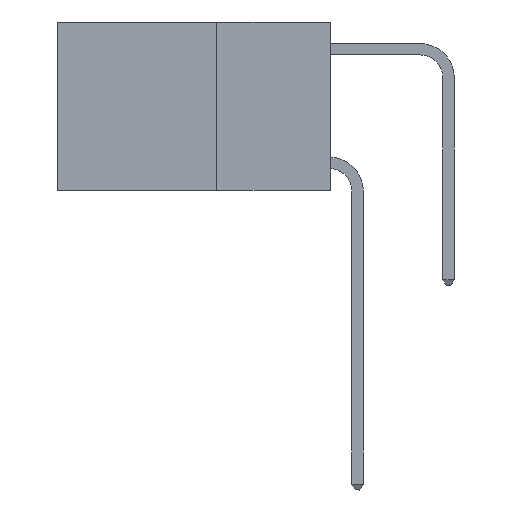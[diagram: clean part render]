
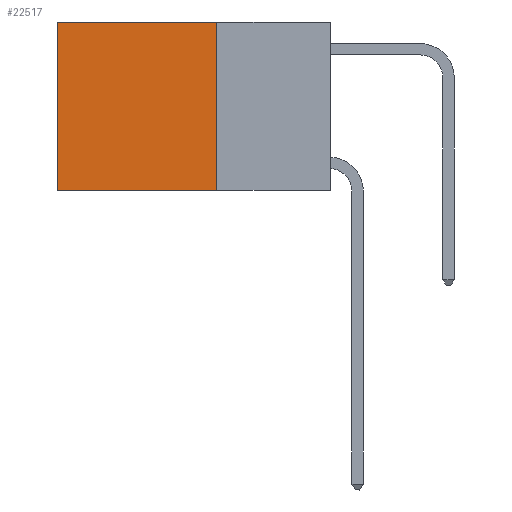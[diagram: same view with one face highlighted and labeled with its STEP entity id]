
A CAD part, left-side view. The second image highlights one B-rep face of the part: STEP entity #22517.
In plain terms, the highlighted planar face has unit normal (-1, 0, 0).
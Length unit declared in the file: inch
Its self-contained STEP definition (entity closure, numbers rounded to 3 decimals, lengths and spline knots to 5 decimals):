
#277 = CARTESIAN_POINT ( 'NONE',  ( 0.2625, 0.6, 0. ) ) ;
#510 = ORIENTED_EDGE ( 'NONE', *, *, #9137, .T. ) ;
#746 = EDGE_CURVE ( 'NONE', #18241, #22927, #17858, .T. ) ;
#994 = ORIENTED_EDGE ( 'NONE', *, *, #746, .F. ) ;
#2169 = DIRECTION ( 'NONE',  ( 0., 0., -1. ) ) ;
#2859 = CARTESIAN_POINT ( 'NONE',  ( 0.2625, 0.25, 0. ) ) ;
#3148 = EDGE_CURVE ( 'NONE', #8559, #22927, #11767, .T. ) ;
#3956 = DIRECTION ( 'NONE',  ( 0., 0., -1. ) ) ;
#4886 = DIRECTION ( 'NONE',  ( 0., 1., 0. ) ) ;
#5256 = CARTESIAN_POINT ( 'NONE',  ( 0.2625, 0.6, 0. ) ) ;
#5821 = CARTESIAN_POINT ( 'NONE',  ( 0.2625, 0.25, 0. ) ) ;
#6109 = CARTESIAN_POINT ( 'NONE',  ( 0.2625, 0.25, 0. ) ) ;
#6649 = AXIS2_PLACEMENT_3D ( 'NONE', #5821, #15421, #3956 ) ;
#8559 = VERTEX_POINT ( 'NONE', #5256 ) ;
#8796 = ORIENTED_EDGE ( 'NONE', *, *, #3148, .T. ) ;
#8860 = CARTESIAN_POINT ( 'NONE',  ( 0.2625, 0.25, 0. ) ) ;
#9137 = EDGE_CURVE ( 'NONE', #9169, #8559, #23282, .T. ) ;
#9169 = VERTEX_POINT ( 'NONE', #8860 ) ;
#9536 = VECTOR ( 'NONE', #21282, 39.37008 ) ;
#10239 = EDGE_CURVE ( 'NONE', #9169, #18241, #15184, .T. ) ;
#10795 = EDGE_LOOP ( 'NONE', ( #8796, #994, #21761, #510 ) ) ;
#11767 = LINE ( 'NONE', #277, #21268 ) ;
#13283 = DIRECTION ( 'NONE',  ( 0., 1., 0. ) ) ;
#13468 = VECTOR ( 'NONE', #13283, 39.37008 ) ;
#13542 = PLANE ( 'NONE',  #6649 ) ;
#15158 = CARTESIAN_POINT ( 'NONE',  ( 0.2625, 0.6, -0.37 ) ) ;
#15184 = LINE ( 'NONE', #6109, #9536 ) ;
#15421 = DIRECTION ( 'NONE',  ( 1., 0., 0. ) ) ;
#17858 = LINE ( 'NONE', #24657, #13468 ) ;
#18171 = VECTOR ( 'NONE', #4886, 39.37008 ) ;
#18241 = VERTEX_POINT ( 'NONE', #20320 ) ;
#19405 = FACE_OUTER_BOUND ( 'NONE', #10795, .T. ) ;
#20320 = CARTESIAN_POINT ( 'NONE',  ( 0.2625, 0.25, -0.37 ) ) ;
#21268 = VECTOR ( 'NONE', #2169, 39.37008 ) ;
#21282 = DIRECTION ( 'NONE',  ( 0., 0., -1. ) ) ;
#21761 = ORIENTED_EDGE ( 'NONE', *, *, #10239, .F. ) ;
#22517 = ADVANCED_FACE ( 'NONE', ( #19405 ), #13542, .F. ) ;
#22927 = VERTEX_POINT ( 'NONE', #15158 ) ;
#23282 = LINE ( 'NONE', #2859, #18171 ) ;
#24657 = CARTESIAN_POINT ( 'NONE',  ( 0.2625, 0.25, -0.37 ) ) ;
